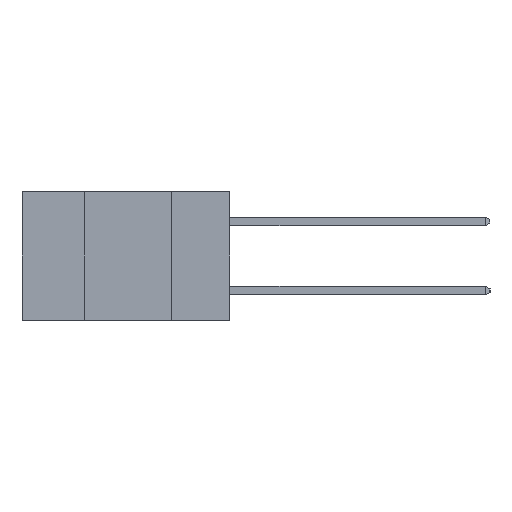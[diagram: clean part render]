
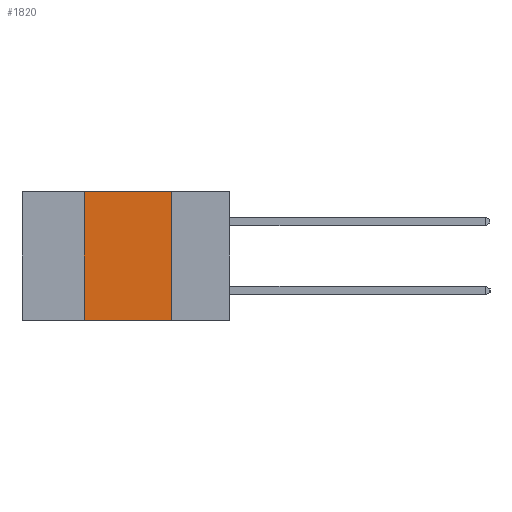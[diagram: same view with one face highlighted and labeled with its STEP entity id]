
A CAD part, left-side view. The second image highlights one B-rep face of the part: STEP entity #1820.
In plain terms, the highlighted planar face has unit normal (-1, 0, 0).
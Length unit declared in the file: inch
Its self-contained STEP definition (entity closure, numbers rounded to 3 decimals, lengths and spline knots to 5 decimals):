
#116 = PLANE ( 'NONE',  #12664 ) ;
#333 = ORIENTED_EDGE ( 'NONE', *, *, #10726, .F. ) ;
#480 = ORIENTED_EDGE ( 'NONE', *, *, #11193, .F. ) ;
#625 = CARTESIAN_POINT ( 'NONE',  ( 0., 0.6, 0. ) ) ;
#799 = CARTESIAN_POINT ( 'NONE',  ( 0., 0.17, 0. ) ) ;
#1285 = CARTESIAN_POINT ( 'NONE',  ( 0., 0.17, -0.37 ) ) ;
#1620 = DIRECTION ( 'NONE',  ( 0., 0., -1. ) ) ;
#1716 = DIRECTION ( 'NONE',  ( 0., 0., -1. ) ) ;
#1793 = ORIENTED_EDGE ( 'NONE', *, *, #2872, .T. ) ;
#1820 = ADVANCED_FACE ( 'NONE', ( #8551 ), #116, .F. ) ;
#2723 = DIRECTION ( 'NONE',  ( 1., 0., 0. ) ) ;
#2872 = EDGE_CURVE ( 'NONE', #6142, #10305, #3514, .T. ) ;
#3514 = LINE ( 'NONE', #11458, #9032 ) ;
#5031 = DIRECTION ( 'NONE',  ( 0., -1., 0. ) ) ;
#5170 = DIRECTION ( 'NONE',  ( 0., 0., 1. ) ) ;
#5216 = CARTESIAN_POINT ( 'NONE',  ( 0., 0.42, -0.37 ) ) ;
#5606 = LINE ( 'NONE', #5216, #5956 ) ;
#5956 = VECTOR ( 'NONE', #5170, 39.37008 ) ;
#6142 = VERTEX_POINT ( 'NONE', #10832 ) ;
#6488 = LINE ( 'NONE', #9075, #12001 ) ;
#6502 = VERTEX_POINT ( 'NONE', #7572 ) ;
#7346 = CARTESIAN_POINT ( 'NONE',  ( 0., 0.17, -0.37 ) ) ;
#7572 = CARTESIAN_POINT ( 'NONE',  ( 0., 0.42, 0. ) ) ;
#7755 = EDGE_LOOP ( 'NONE', ( #480, #333, #8110, #1793 ) ) ;
#8110 = ORIENTED_EDGE ( 'NONE', *, *, #11734, .F. ) ;
#8551 = FACE_OUTER_BOUND ( 'NONE', #7755, .T. ) ;
#8758 = VECTOR ( 'NONE', #1716, 39.37008 ) ;
#9032 = VECTOR ( 'NONE', #5031, 39.37008 ) ;
#9038 = DIRECTION ( 'NONE',  ( 0., -1., 0. ) ) ;
#9075 = CARTESIAN_POINT ( 'NONE',  ( 0., 0.6, 0. ) ) ;
#10305 = VERTEX_POINT ( 'NONE', #7346 ) ;
#10726 = EDGE_CURVE ( 'NONE', #6502, #12011, #6488, .T. ) ;
#10832 = CARTESIAN_POINT ( 'NONE',  ( 0., 0.42, -0.37 ) ) ;
#11193 = EDGE_CURVE ( 'NONE', #12011, #10305, #11649, .T. ) ;
#11458 = CARTESIAN_POINT ( 'NONE',  ( 0., 0.6, -0.37 ) ) ;
#11649 = LINE ( 'NONE', #1285, #8758 ) ;
#11734 = EDGE_CURVE ( 'NONE', #6142, #6502, #5606, .T. ) ;
#12001 = VECTOR ( 'NONE', #9038, 39.37008 ) ;
#12011 = VERTEX_POINT ( 'NONE', #799 ) ;
#12664 = AXIS2_PLACEMENT_3D ( 'NONE', #625, #2723, #1620 ) ;
